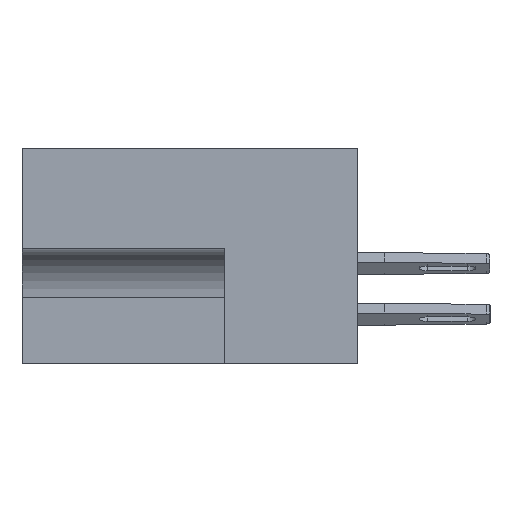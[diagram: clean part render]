
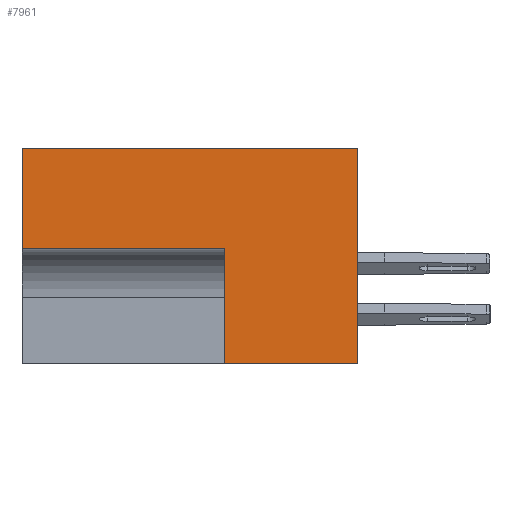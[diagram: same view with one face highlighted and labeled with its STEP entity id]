
A CAD part, left-side view. The second image highlights one B-rep face of the part: STEP entity #7961.
In plain terms, the highlighted planar face has unit normal (-1, 0, 0).
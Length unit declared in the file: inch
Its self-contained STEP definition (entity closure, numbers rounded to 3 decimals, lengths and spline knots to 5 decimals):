
#635 = LINE ( 'NONE', #20536, #10997 ) ;
#1070 = CARTESIAN_POINT ( 'NONE',  ( 0., 0.328, -0.248 ) ) ;
#2006 = CARTESIAN_POINT ( 'NONE',  ( 0., 0.828, -0.248 ) ) ;
#2024 = DIRECTION ( 'NONE',  ( 0., -1., 0. ) ) ;
#2626 = VERTEX_POINT ( 'NONE', #25036 ) ;
#3771 = CARTESIAN_POINT ( 'NONE',  ( 0., 0.328, -0.531 ) ) ;
#4209 = DIRECTION ( 'NONE',  ( 0., 1., 0. ) ) ;
#4311 = CARTESIAN_POINT ( 'NONE',  ( 0., 0.453, -0.531 ) ) ;
#5169 = VECTOR ( 'NONE', #22368, 39.37008 ) ;
#5253 = DIRECTION ( 'NONE',  ( 0., 0., -1. ) ) ;
#6581 = VERTEX_POINT ( 'NONE', #9280 ) ;
#6778 = LINE ( 'NONE', #23977, #21577 ) ;
#7290 = ORIENTED_EDGE ( 'NONE', *, *, #15606, .F. ) ;
#7621 = CARTESIAN_POINT ( 'NONE',  ( 0., 0.453, 0. ) ) ;
#7961 = ADVANCED_FACE ( 'NONE', ( #16212 ), #19181, .F. ) ;
#8172 = LINE ( 'NONE', #15892, #29995 ) ;
#8483 = VERTEX_POINT ( 'NONE', #1070 ) ;
#8484 = LINE ( 'NONE', #27209, #5169 ) ;
#9280 = CARTESIAN_POINT ( 'NONE',  ( 0., 0., 0. ) ) ;
#9374 = EDGE_CURVE ( 'NONE', #28803, #2626, #21763, .T. ) ;
#10311 = VERTEX_POINT ( 'NONE', #23009 ) ;
#10997 = VECTOR ( 'NONE', #4209, 39.37008 ) ;
#11843 = EDGE_CURVE ( 'NONE', #10311, #6581, #6778, .T. ) ;
#15507 = VECTOR ( 'NONE', #27442, 39.37008 ) ;
#15606 = EDGE_CURVE ( 'NONE', #23938, #10311, #8484, .T. ) ;
#15892 = CARTESIAN_POINT ( 'NONE',  ( 0., 0., 0. ) ) ;
#16212 = FACE_OUTER_BOUND ( 'NONE', #18134, .T. ) ;
#16403 = EDGE_CURVE ( 'NONE', #8483, #23938, #635, .T. ) ;
#16958 = ORIENTED_EDGE ( 'NONE', *, *, #11843, .F. ) ;
#17115 = ORIENTED_EDGE ( 'NONE', *, *, #28015, .F. ) ;
#18134 = EDGE_LOOP ( 'NONE', ( #7290, #25955, #17115, #28646, #29705, #16958 ) ) ;
#19181 = PLANE ( 'NONE',  #19230 ) ;
#19230 = AXIS2_PLACEMENT_3D ( 'NONE', #7621, #21375, #5253 ) ;
#20536 = CARTESIAN_POINT ( 'NONE',  ( 0., 0.328, -0.248 ) ) ;
#21375 = DIRECTION ( 'NONE',  ( 1., 0., 0. ) ) ;
#21577 = VECTOR ( 'NONE', #28421, 39.37008 ) ;
#21763 = LINE ( 'NONE', #4311, #23243 ) ;
#21836 = LINE ( 'NONE', #3771, #15507 ) ;
#22368 = DIRECTION ( 'NONE',  ( 0., 0., 1. ) ) ;
#23009 = CARTESIAN_POINT ( 'NONE',  ( 0., 0.828, 0. ) ) ;
#23243 = VECTOR ( 'NONE', #2024, 39.37008 ) ;
#23477 = CARTESIAN_POINT ( 'NONE',  ( 0., 0.328, -0.531 ) ) ;
#23938 = VERTEX_POINT ( 'NONE', #2006 ) ;
#23977 = CARTESIAN_POINT ( 'NONE',  ( 0., 0.453, 0. ) ) ;
#25036 = CARTESIAN_POINT ( 'NONE',  ( 0., 0., -0.531 ) ) ;
#25955 = ORIENTED_EDGE ( 'NONE', *, *, #16403, .F. ) ;
#27209 = CARTESIAN_POINT ( 'NONE',  ( 0., 0.828, 0. ) ) ;
#27366 = EDGE_CURVE ( 'NONE', #2626, #6581, #8172, .T. ) ;
#27442 = DIRECTION ( 'NONE',  ( 0., 0., 1. ) ) ;
#28015 = EDGE_CURVE ( 'NONE', #28803, #8483, #21836, .T. ) ;
#28421 = DIRECTION ( 'NONE',  ( 0., -1., 0. ) ) ;
#28646 = ORIENTED_EDGE ( 'NONE', *, *, #9374, .T. ) ;
#28803 = VERTEX_POINT ( 'NONE', #23477 ) ;
#29705 = ORIENTED_EDGE ( 'NONE', *, *, #27366, .T. ) ;
#29854 = DIRECTION ( 'NONE',  ( 0., 0., 1. ) ) ;
#29995 = VECTOR ( 'NONE', #29854, 39.37008 ) ;
